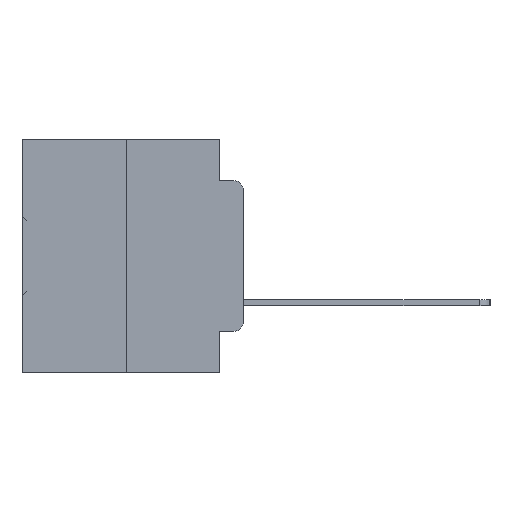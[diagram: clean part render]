
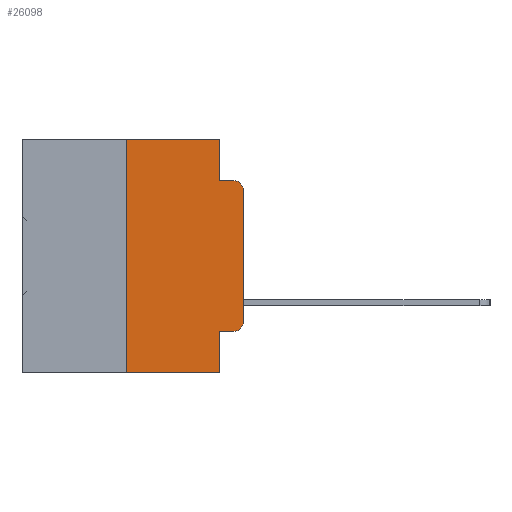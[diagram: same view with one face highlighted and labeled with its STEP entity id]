
A CAD part, left-side view. The second image highlights one B-rep face of the part: STEP entity #26098.
In plain terms, the highlighted planar face has unit normal (-1, 0, 0).
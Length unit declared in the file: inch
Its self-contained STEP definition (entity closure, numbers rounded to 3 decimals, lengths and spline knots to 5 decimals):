
#681 = LINE ( 'NONE', #7729, #5594 ) ;
#854 = EDGE_CURVE ( 'NONE', #1723, #36325, #31865, .T. ) ;
#896 = CARTESIAN_POINT ( 'NONE',  ( 0., 0.051, 0. ) ) ;
#1225 = ORIENTED_EDGE ( 'NONE', *, *, #23519, .T. ) ;
#1270 = EDGE_LOOP ( 'NONE', ( #6227, #29650, #23147, #1304, #10745, #33102, #3474, #18652, #21323, #1225 ) ) ;
#1304 = ORIENTED_EDGE ( 'NONE', *, *, #30722, .F. ) ;
#1515 = DIRECTION ( 'NONE',  ( 0., -1., 0. ) ) ;
#1723 = VERTEX_POINT ( 'NONE', #30384 ) ;
#2203 = AXIS2_PLACEMENT_3D ( 'NONE', #31387, #14627, #34149 ) ;
#2216 = VERTEX_POINT ( 'NONE', #15238 ) ;
#3474 = ORIENTED_EDGE ( 'NONE', *, *, #31456, .T. ) ;
#3494 = LINE ( 'NONE', #15878, #17794 ) ;
#3565 = LINE ( 'NONE', #896, #30083 ) ;
#5045 = CARTESIAN_POINT ( 'NONE',  ( 0., 0.051, -0.4115 ) ) ;
#5411 = EDGE_CURVE ( 'NONE', #2216, #9565, #5780, .T. ) ;
#5594 = VECTOR ( 'NONE', #16355, 39.37008 ) ;
#5780 = LINE ( 'NONE', #18617, #20971 ) ;
#6227 = ORIENTED_EDGE ( 'NONE', *, *, #854, .T. ) ;
#7352 = EDGE_CURVE ( 'NONE', #36325, #9565, #35928, .T. ) ;
#7729 = CARTESIAN_POINT ( 'NONE',  ( 0., 0.051, 0. ) ) ;
#7965 = CARTESIAN_POINT ( 'NONE',  ( 0., 0.02, -0.0885 ) ) ;
#8120 = VECTOR ( 'NONE', #10801, 39.37008 ) ;
#8245 = PLANE ( 'NONE',  #32533 ) ;
#9013 = LINE ( 'NONE', #30333, #8120 ) ;
#9565 = VERTEX_POINT ( 'NONE', #7965 ) ;
#10745 = ORIENTED_EDGE ( 'NONE', *, *, #20611, .F. ) ;
#10801 = DIRECTION ( 'NONE',  ( 0., 0., 1. ) ) ;
#11158 = DIRECTION ( 'NONE',  ( 1., 0., 0. ) ) ;
#11789 = DIRECTION ( 'NONE',  ( 0., -1., 0. ) ) ;
#12180 = VECTOR ( 'NONE', #11789, 39.37008 ) ;
#12344 = VERTEX_POINT ( 'NONE', #18509 ) ;
#12817 = VERTEX_POINT ( 'NONE', #18238 ) ;
#13088 = LINE ( 'NONE', #20234, #12180 ) ;
#13284 = DIRECTION ( 'NONE',  ( -1., 0., 0. ) ) ;
#13390 = DIRECTION ( 'NONE',  ( 0., 0., 1. ) ) ;
#14520 = LINE ( 'NONE', #5045, #20299 ) ;
#14627 = DIRECTION ( 'NONE',  ( -1., 0., 0. ) ) ;
#14957 = CARTESIAN_POINT ( 'NONE',  ( 0., 0.051, 0. ) ) ;
#15238 = CARTESIAN_POINT ( 'NONE',  ( 0., 0.051, -0.0885 ) ) ;
#15878 = CARTESIAN_POINT ( 'NONE',  ( 0., 0.473, -0.5 ) ) ;
#16355 = DIRECTION ( 'NONE',  ( 0., 0., -1. ) ) ;
#17794 = VECTOR ( 'NONE', #18713, 39.37008 ) ;
#17883 = VERTEX_POINT ( 'NONE', #30003 ) ;
#18238 = CARTESIAN_POINT ( 'NONE',  ( 0., 0.25, 0. ) ) ;
#18277 = AXIS2_PLACEMENT_3D ( 'NONE', #30065, #13284, #32837 ) ;
#18509 = CARTESIAN_POINT ( 'NONE',  ( 0., 0.051, -0.4115 ) ) ;
#18617 = CARTESIAN_POINT ( 'NONE',  ( 0., 0.051, -0.0885 ) ) ;
#18652 = ORIENTED_EDGE ( 'NONE', *, *, #26524, .F. ) ;
#18713 = DIRECTION ( 'NONE',  ( 0., -1., 0. ) ) ;
#19548 = VERTEX_POINT ( 'NONE', #14957 ) ;
#19598 = CARTESIAN_POINT ( 'NONE',  ( 0., 0.473, 0. ) ) ;
#19982 = CARTESIAN_POINT ( 'NONE',  ( 0., 0., 0. ) ) ;
#20234 = CARTESIAN_POINT ( 'NONE',  ( 0., 0.473, 0. ) ) ;
#20299 = VECTOR ( 'NONE', #24898, 39.37008 ) ;
#20611 = EDGE_CURVE ( 'NONE', #12817, #19548, #13088, .T. ) ;
#20971 = VECTOR ( 'NONE', #1515, 39.37008 ) ;
#21323 = ORIENTED_EDGE ( 'NONE', *, *, #27208, .T. ) ;
#22637 = CARTESIAN_POINT ( 'NONE',  ( 0., 0.051, -0.5 ) ) ;
#23147 = ORIENTED_EDGE ( 'NONE', *, *, #5411, .F. ) ;
#23300 = EDGE_CURVE ( 'NONE', #33045, #12817, #9013, .T. ) ;
#23519 = EDGE_CURVE ( 'NONE', #17883, #1723, #31013, .T. ) ;
#23652 = VECTOR ( 'NONE', #13390, 39.37008 ) ;
#23703 = DIRECTION ( 'NONE',  ( 0., 0., -1. ) ) ;
#24898 = DIRECTION ( 'NONE',  ( 0., -1., 0. ) ) ;
#26098 = ADVANCED_FACE ( 'NONE', ( #28209 ), #8245, .F. ) ;
#26524 = EDGE_CURVE ( 'NONE', #12344, #28600, #681, .T. ) ;
#27208 = EDGE_CURVE ( 'NONE', #12344, #17883, #14520, .T. ) ;
#28209 = FACE_OUTER_BOUND ( 'NONE', #1270, .T. ) ;
#28600 = VERTEX_POINT ( 'NONE', #22637 ) ;
#29650 = ORIENTED_EDGE ( 'NONE', *, *, #7352, .T. ) ;
#30003 = CARTESIAN_POINT ( 'NONE',  ( 0., 0.02, -0.4115 ) ) ;
#30065 = CARTESIAN_POINT ( 'NONE',  ( 0., 0.02, -0.1085 ) ) ;
#30083 = VECTOR ( 'NONE', #23703, 39.37008 ) ;
#30333 = CARTESIAN_POINT ( 'NONE',  ( 0., 0.25, 0. ) ) ;
#30384 = CARTESIAN_POINT ( 'NONE',  ( 0., 0., -0.3915 ) ) ;
#30700 = CARTESIAN_POINT ( 'NONE',  ( 0., 0., -0.1085 ) ) ;
#30722 = EDGE_CURVE ( 'NONE', #19548, #2216, #3565, .T. ) ;
#30790 = DIRECTION ( 'NONE',  ( 0., 0., -1. ) ) ;
#31013 = CIRCLE ( 'NONE', #2203, 0.02 ) ;
#31387 = CARTESIAN_POINT ( 'NONE',  ( 0., 0.02, -0.3915 ) ) ;
#31456 = EDGE_CURVE ( 'NONE', #33045, #28600, #3494, .T. ) ;
#31865 = LINE ( 'NONE', #19982, #23652 ) ;
#31888 = CARTESIAN_POINT ( 'NONE',  ( 0., 0.25, -0.5 ) ) ;
#32533 = AXIS2_PLACEMENT_3D ( 'NONE', #19598, #11158, #30790 ) ;
#32837 = DIRECTION ( 'NONE',  ( 0., 0., -1. ) ) ;
#33045 = VERTEX_POINT ( 'NONE', #31888 ) ;
#33102 = ORIENTED_EDGE ( 'NONE', *, *, #23300, .F. ) ;
#34149 = DIRECTION ( 'NONE',  ( 0., 0., -1. ) ) ;
#35928 = CIRCLE ( 'NONE', #18277, 0.02 ) ;
#36325 = VERTEX_POINT ( 'NONE', #30700 ) ;
